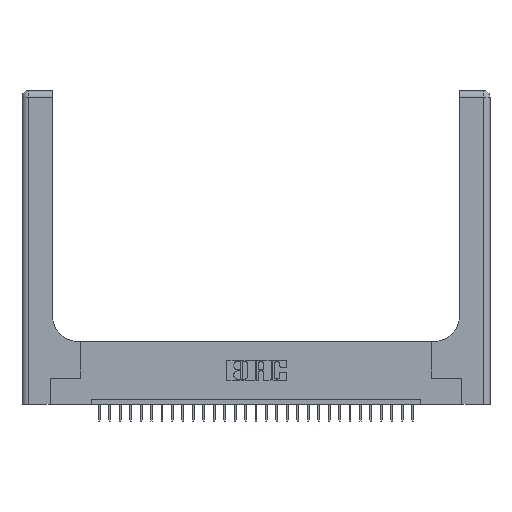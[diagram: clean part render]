
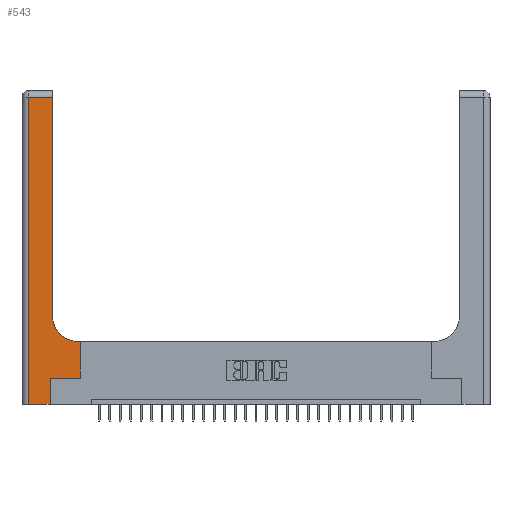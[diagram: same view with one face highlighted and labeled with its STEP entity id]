
A CAD part, top view. The second image highlights one B-rep face of the part: STEP entity #543.
In plain terms, the highlighted planar face has unit normal (0, 0, 1).
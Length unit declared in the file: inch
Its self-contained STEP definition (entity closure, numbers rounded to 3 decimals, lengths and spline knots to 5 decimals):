
#361 = EDGE_CURVE ( 'NONE', #6552, #23287, #4649, .T. ) ;
#543 = ADVANCED_FACE ( 'NONE', ( #22490 ), #552, .F. ) ;
#552 = PLANE ( 'NONE',  #25917 ) ;
#649 = CARTESIAN_POINT ( 'NONE',  ( 0.269, 0.25, 0.37 ) ) ;
#1067 = ORIENTED_EDGE ( 'NONE', *, *, #12912, .T. ) ;
#1649 = EDGE_CURVE ( 'NONE', #20702, #6552, #22810, .T. ) ;
#2996 = CARTESIAN_POINT ( 'NONE',  ( 0., 3., 0.37 ) ) ;
#3020 = VERTEX_POINT ( 'NONE', #22502 ) ;
#3315 = DIRECTION ( 'NONE',  ( -1., 0., 0. ) ) ;
#3812 = EDGE_CURVE ( 'NONE', #23822, #25438, #13116, .T. ) ;
#3927 = DIRECTION ( 'NONE',  ( 0., 0., -1. ) ) ;
#4649 = LINE ( 'NONE', #22074, #11573 ) ;
#5713 = CARTESIAN_POINT ( 'NONE',  ( 0.06, 2.94, 0.37 ) ) ;
#6429 = DIRECTION ( 'NONE',  ( 1., 0., 0. ) ) ;
#6537 = CARTESIAN_POINT ( 'NONE',  ( 0., 0., 0.37 ) ) ;
#6552 = VERTEX_POINT ( 'NONE', #21893 ) ;
#6923 = CIRCLE ( 'NONE', #9404, 0.25 ) ;
#7092 = ORIENTED_EDGE ( 'NONE', *, *, #20831, .T. ) ;
#7159 = CARTESIAN_POINT ( 'NONE',  ( 0.2915, 0.85, 0.37 ) ) ;
#7371 = ORIENTED_EDGE ( 'NONE', *, *, #8594, .T. ) ;
#7634 = VECTOR ( 'NONE', #6429, 39.37008 ) ;
#8214 = CARTESIAN_POINT ( 'NONE',  ( 0.2915, 3., 0.37 ) ) ;
#8245 = CARTESIAN_POINT ( 'NONE',  ( 0.269, 0., 0.37 ) ) ;
#8594 = EDGE_CURVE ( 'NONE', #23287, #28746, #24216, .T. ) ;
#9114 = LINE ( 'NONE', #6537, #7634 ) ;
#9404 = AXIS2_PLACEMENT_3D ( 'NONE', #28487, #3927, #23112 ) ;
#10871 = CARTESIAN_POINT ( 'NONE',  ( 0.2915, 0.6, 0.37 ) ) ;
#11237 = DIRECTION ( 'NONE',  ( 0., 1., 0. ) ) ;
#11568 = CARTESIAN_POINT ( 'NONE',  ( 0.5415, 0.6, 0.37 ) ) ;
#11573 = VECTOR ( 'NONE', #3315, 39.37008 ) ;
#12146 = CARTESIAN_POINT ( 'NONE',  ( 0.06, 3., 0.37 ) ) ;
#12457 = DIRECTION ( 'NONE',  ( 1., 0., 0. ) ) ;
#12483 = DIRECTION ( 'NONE',  ( 0., 1., 0. ) ) ;
#12912 = EDGE_CURVE ( 'NONE', #25438, #20702, #6923, .T. ) ;
#13116 = LINE ( 'NONE', #10871, #20356 ) ;
#13135 = CARTESIAN_POINT ( 'NONE',  ( 0.5585, 0.6, 0.37 ) ) ;
#13768 = VERTEX_POINT ( 'NONE', #16728 ) ;
#14084 = VECTOR ( 'NONE', #12483, 39.37008 ) ;
#14185 = DIRECTION ( 'NONE',  ( -1., 0., 0. ) ) ;
#14207 = ORIENTED_EDGE ( 'NONE', *, *, #26594, .T. ) ;
#14915 = ORIENTED_EDGE ( 'NONE', *, *, #22614, .T. ) ;
#14937 = VECTOR ( 'NONE', #12457, 39.37008 ) ;
#16097 = EDGE_LOOP ( 'NONE', ( #18016, #27909, #7371, #14207, #23953, #7092, #14915, #21328, #1067 ) ) ;
#16539 = LINE ( 'NONE', #24763, #24913 ) ;
#16728 = CARTESIAN_POINT ( 'NONE',  ( 0.5585, 0.25, 0.37 ) ) ;
#17472 = LINE ( 'NONE', #649, #14937 ) ;
#18016 = ORIENTED_EDGE ( 'NONE', *, *, #1649, .T. ) ;
#18084 = VECTOR ( 'NONE', #11237, 39.37008 ) ;
#19917 = DIRECTION ( 'NONE',  ( -1., 0., 0. ) ) ;
#20311 = DIRECTION ( 'NONE',  ( 0., 1., 0. ) ) ;
#20356 = VECTOR ( 'NONE', #19917, 39.37008 ) ;
#20366 = CARTESIAN_POINT ( 'NONE',  ( 0.06, 0., 0.37 ) ) ;
#20612 = VECTOR ( 'NONE', #24427, 39.37008 ) ;
#20702 = VERTEX_POINT ( 'NONE', #7159 ) ;
#20831 = EDGE_CURVE ( 'NONE', #3020, #13768, #17472, .T. ) ;
#20989 = LINE ( 'NONE', #24041, #14084 ) ;
#21328 = ORIENTED_EDGE ( 'NONE', *, *, #3812, .T. ) ;
#21893 = CARTESIAN_POINT ( 'NONE',  ( 0.2915, 2.94, 0.37 ) ) ;
#22074 = CARTESIAN_POINT ( 'NONE',  ( 0., 2.94, 0.37 ) ) ;
#22490 = FACE_OUTER_BOUND ( 'NONE', #16097, .T. ) ;
#22502 = CARTESIAN_POINT ( 'NONE',  ( 0.269, 0.25, 0.37 ) ) ;
#22614 = EDGE_CURVE ( 'NONE', #13768, #23822, #20989, .T. ) ;
#22810 = LINE ( 'NONE', #8214, #18084 ) ;
#23112 = DIRECTION ( 'NONE',  ( 1., 0., 0. ) ) ;
#23287 = VERTEX_POINT ( 'NONE', #5713 ) ;
#23822 = VERTEX_POINT ( 'NONE', #13135 ) ;
#23953 = ORIENTED_EDGE ( 'NONE', *, *, #29745, .T. ) ;
#24041 = CARTESIAN_POINT ( 'NONE',  ( 0.5585, 0.25, 0.37 ) ) ;
#24216 = LINE ( 'NONE', #12146, #20612 ) ;
#24427 = DIRECTION ( 'NONE',  ( 0., -1., 0. ) ) ;
#24763 = CARTESIAN_POINT ( 'NONE',  ( 0.269, 0., 0.37 ) ) ;
#24913 = VECTOR ( 'NONE', #20311, 39.37008 ) ;
#25130 = VERTEX_POINT ( 'NONE', #8245 ) ;
#25438 = VERTEX_POINT ( 'NONE', #11568 ) ;
#25917 = AXIS2_PLACEMENT_3D ( 'NONE', #2996, #28189, #14185 ) ;
#26594 = EDGE_CURVE ( 'NONE', #28746, #25130, #9114, .T. ) ;
#27909 = ORIENTED_EDGE ( 'NONE', *, *, #361, .T. ) ;
#28189 = DIRECTION ( 'NONE',  ( 0., 0., -1. ) ) ;
#28487 = CARTESIAN_POINT ( 'NONE',  ( 0.5415, 0.85, 0.37 ) ) ;
#28746 = VERTEX_POINT ( 'NONE', #20366 ) ;
#29745 = EDGE_CURVE ( 'NONE', #25130, #3020, #16539, .T. ) ;
